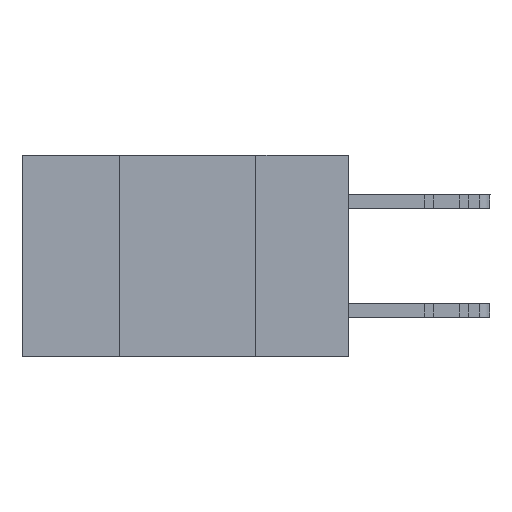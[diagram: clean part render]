
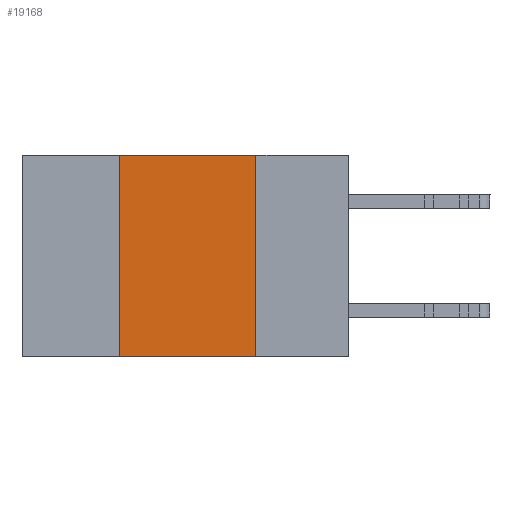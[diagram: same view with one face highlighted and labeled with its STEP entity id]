
A CAD part, left-side view. The second image highlights one B-rep face of the part: STEP entity #19168.
In plain terms, the highlighted planar face has unit normal (-1, 0, 0).
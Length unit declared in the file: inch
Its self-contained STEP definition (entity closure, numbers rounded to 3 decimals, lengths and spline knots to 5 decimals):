
#791 = VECTOR ( 'NONE', #4659, 39.37008 ) ;
#1976 = CARTESIAN_POINT ( 'NONE',  ( 0., 0.42, 0. ) ) ;
#2426 = LINE ( 'NONE', #26377, #17592 ) ;
#4659 = DIRECTION ( 'NONE',  ( 0., -1., 0. ) ) ;
#4977 = EDGE_CURVE ( 'NONE', #12279, #33506, #13907, .T. ) ;
#5002 = DIRECTION ( 'NONE',  ( 0., 0., -1. ) ) ;
#5358 = CARTESIAN_POINT ( 'NONE',  ( 0., 0.42, -0.37 ) ) ;
#7236 = LINE ( 'NONE', #1976, #11460 ) ;
#7849 = DIRECTION ( 'NONE',  ( 0., -1., 0. ) ) ;
#10823 = EDGE_CURVE ( 'NONE', #22144, #33506, #20547, .T. ) ;
#11460 = VECTOR ( 'NONE', #23621, 39.37008 ) ;
#12279 = VERTEX_POINT ( 'NONE', #14825 ) ;
#13907 = LINE ( 'NONE', #32588, #25733 ) ;
#14825 = CARTESIAN_POINT ( 'NONE',  ( 0., 0.17, 0. ) ) ;
#15467 = ORIENTED_EDGE ( 'NONE', *, *, #31342, .F. ) ;
#15999 = EDGE_CURVE ( 'NONE', #22144, #22766, #7236, .T. ) ;
#17476 = ORIENTED_EDGE ( 'NONE', *, *, #4977, .F. ) ;
#17592 = VECTOR ( 'NONE', #7849, 39.37008 ) ;
#19168 = ADVANCED_FACE ( 'NONE', ( #23509 ), #34002, .F. ) ;
#20547 = LINE ( 'NONE', #31036, #791 ) ;
#20656 = CARTESIAN_POINT ( 'NONE',  ( 0., 0.42, 0. ) ) ;
#21935 = EDGE_LOOP ( 'NONE', ( #17476, #15467, #25960, #27846 ) ) ;
#22144 = VERTEX_POINT ( 'NONE', #5358 ) ;
#22766 = VERTEX_POINT ( 'NONE', #20656 ) ;
#23509 = FACE_OUTER_BOUND ( 'NONE', #21935, .T. ) ;
#23621 = DIRECTION ( 'NONE',  ( 0., 0., 1. ) ) ;
#25733 = VECTOR ( 'NONE', #27894, 39.37008 ) ;
#25960 = ORIENTED_EDGE ( 'NONE', *, *, #15999, .F. ) ;
#26377 = CARTESIAN_POINT ( 'NONE',  ( 0., 0.6, 0. ) ) ;
#27846 = ORIENTED_EDGE ( 'NONE', *, *, #10823, .T. ) ;
#27894 = DIRECTION ( 'NONE',  ( 0., 0., -1. ) ) ;
#31001 = CARTESIAN_POINT ( 'NONE',  ( 0., 0.17, -0.37 ) ) ;
#31036 = CARTESIAN_POINT ( 'NONE',  ( 0., 0.6, -0.37 ) ) ;
#31342 = EDGE_CURVE ( 'NONE', #22766, #12279, #2426, .T. ) ;
#31549 = DIRECTION ( 'NONE',  ( 1., 0., 0. ) ) ;
#32588 = CARTESIAN_POINT ( 'NONE',  ( 0., 0.17, 0. ) ) ;
#33506 = VERTEX_POINT ( 'NONE', #31001 ) ;
#33933 = AXIS2_PLACEMENT_3D ( 'NONE', #34167, #31549, #5002 ) ;
#34002 = PLANE ( 'NONE',  #33933 ) ;
#34167 = CARTESIAN_POINT ( 'NONE',  ( 0., 0.6, 0. ) ) ;
